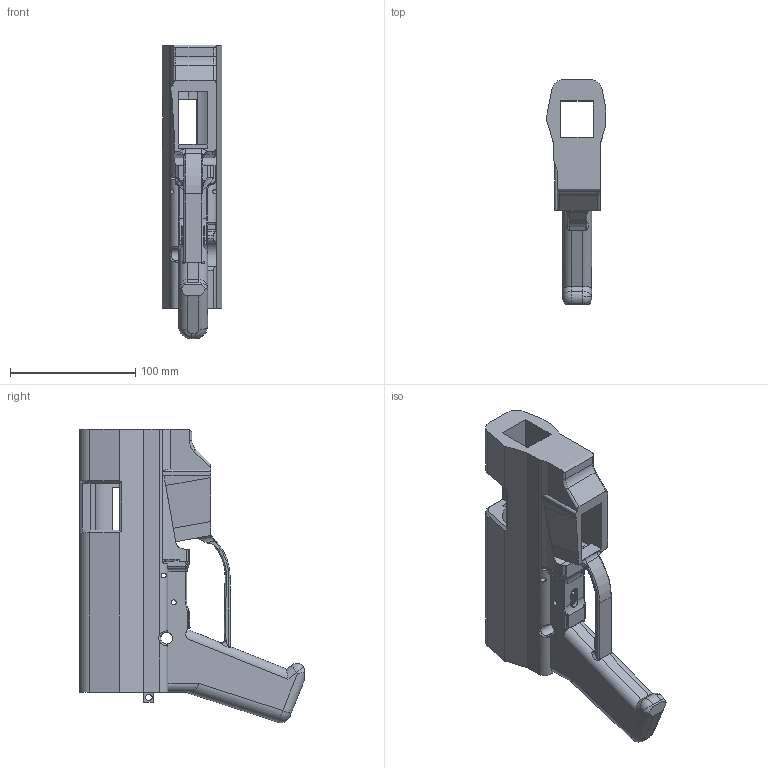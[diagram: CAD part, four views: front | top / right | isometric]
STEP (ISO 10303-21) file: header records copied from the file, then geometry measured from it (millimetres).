
FILE_DESCRIPTION (( 'STEP AP214' ), '1' );
FILE_NAME ('Receiver.STEP', '2013-11-06T01:45:56', ( '' ), ( '' ), 'SwSTEP 2.0', 'SolidWorks 2013', '' );
FILE_SCHEMA (( 'AUTOMOTIVE_DESIGN' ));
Length unit declared in the file: millimetre
Products named in the file (1): Receiver
Bounding box: 47.55 x 179.26 x 233.9 mm (x, y, z)
Volume: 478794 mm3; surface area: 109959 mm2
Topology: 1 solids, 1 shells, 340 faces, 958 edges, 604 vertices
Faces by surface type: plane 135, cylinder 132, bspline 43, torus 20, sphere 6, cone 4
Entity records: 15096 total; most frequent: CARTESIAN_POINT 6771, ORIENTED_EDGE 1898, DIRECTION 1549, EDGE_CURVE 949, VERTEX_POINT 602, AXIS2_PLACEMENT_3D 523, LINE 503, VECTOR 503
